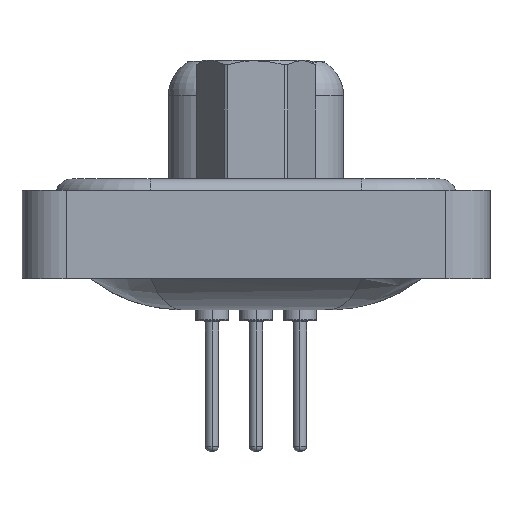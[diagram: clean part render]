
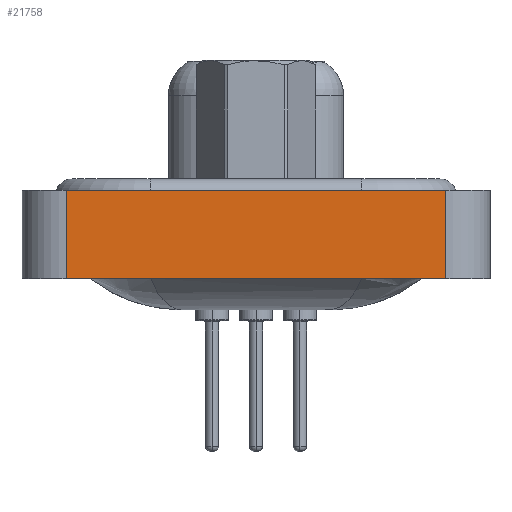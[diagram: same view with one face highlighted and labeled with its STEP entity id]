
A CAD part, left-side view. The second image highlights one B-rep face of the part: STEP entity #21758.
In plain terms, the highlighted planar face has unit normal (-1, 0, 0).
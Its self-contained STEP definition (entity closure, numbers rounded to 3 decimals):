
#678 = VECTOR ( 'NONE', #15960, 1000. ) ;
#1291 = LINE ( 'NONE', #10016, #678 ) ;
#1874 = CARTESIAN_POINT ( 'NONE',  ( -7.26, 8.55, -3.6 ) ) ;
#3406 = CARTESIAN_POINT ( 'NONE',  ( -7.26, -8.55, 0.4 ) ) ;
#4433 = EDGE_LOOP ( 'NONE', ( #11015, #24292, #7940, #5209 ) ) ;
#5209 = ORIENTED_EDGE ( 'NONE', *, *, #14824, .T. ) ;
#5430 = FACE_OUTER_BOUND ( 'NONE', #4433, .T. ) ;
#5960 = CARTESIAN_POINT ( 'NONE',  ( -7.26, 8.55, 0.4 ) ) ;
#6204 = EDGE_CURVE ( 'NONE', #22670, #11831, #8378, .T. ) ;
#7940 = ORIENTED_EDGE ( 'NONE', *, *, #6204, .F. ) ;
#8378 = LINE ( 'NONE', #9333, #20102 ) ;
#8558 = LINE ( 'NONE', #11828, #23686 ) ;
#8590 = CARTESIAN_POINT ( 'NONE',  ( -7.26, -8.55, 0.4 ) ) ;
#9333 = CARTESIAN_POINT ( 'NONE',  ( -7.26, 8.55, -3.6 ) ) ;
#9822 = DIRECTION ( 'NONE',  ( 0., 0., 1. ) ) ;
#10016 = CARTESIAN_POINT ( 'NONE',  ( -7.26, -8.55, -3.6 ) ) ;
#11015 = ORIENTED_EDGE ( 'NONE', *, *, #20023, .T. ) ;
#11196 = AXIS2_PLACEMENT_3D ( 'NONE', #12490, #24415, #12568 ) ;
#11828 = CARTESIAN_POINT ( 'NONE',  ( -7.26, -8.55, -3.6 ) ) ;
#11831 = VERTEX_POINT ( 'NONE', #5960 ) ;
#12490 = CARTESIAN_POINT ( 'NONE',  ( -7.26, -8.55, -3.6 ) ) ;
#12568 = DIRECTION ( 'NONE',  ( 0., 0., 1. ) ) ;
#14280 = EDGE_CURVE ( 'NONE', #11831, #20953, #14626, .T. ) ;
#14626 = LINE ( 'NONE', #3406, #24532 ) ;
#14824 = EDGE_CURVE ( 'NONE', #22670, #21308, #1291, .T. ) ;
#15170 = CARTESIAN_POINT ( 'NONE',  ( -7.26, -8.55, -3.6 ) ) ;
#15960 = DIRECTION ( 'NONE',  ( 0., -1., 0. ) ) ;
#16921 = DIRECTION ( 'NONE',  ( 0., 0., 1. ) ) ;
#20023 = EDGE_CURVE ( 'NONE', #21308, #20953, #8558, .T. ) ;
#20102 = VECTOR ( 'NONE', #16921, 1000. ) ;
#20953 = VERTEX_POINT ( 'NONE', #8590 ) ;
#21308 = VERTEX_POINT ( 'NONE', #15170 ) ;
#21758 = ADVANCED_FACE ( 'NONE', ( #5430 ), #22404, .T. ) ;
#22404 = PLANE ( 'NONE',  #11196 ) ;
#22670 = VERTEX_POINT ( 'NONE', #1874 ) ;
#23686 = VECTOR ( 'NONE', #9822, 1000. ) ;
#24292 = ORIENTED_EDGE ( 'NONE', *, *, #14280, .F. ) ;
#24415 = DIRECTION ( 'NONE',  ( -1., 0., 0. ) ) ;
#24532 = VECTOR ( 'NONE', #25101, 1000. ) ;
#25101 = DIRECTION ( 'NONE',  ( 0., -1., 0. ) ) ;
